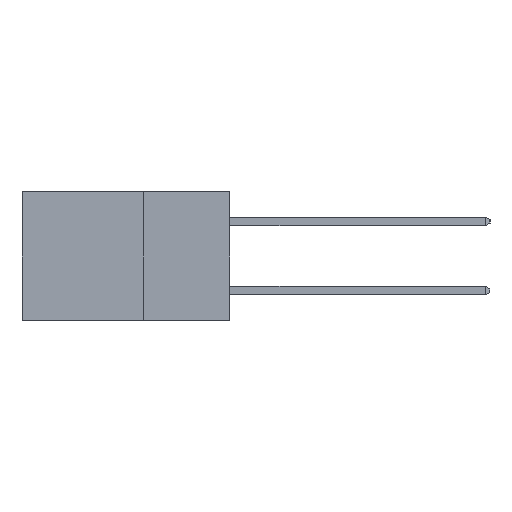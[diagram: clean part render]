
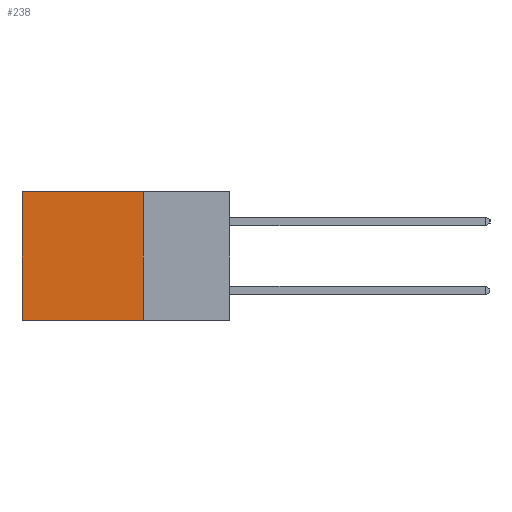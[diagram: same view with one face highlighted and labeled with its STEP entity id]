
A CAD part, left-side view. The second image highlights one B-rep face of the part: STEP entity #238.
In plain terms, the highlighted planar face has unit normal (-1, 0, 0).
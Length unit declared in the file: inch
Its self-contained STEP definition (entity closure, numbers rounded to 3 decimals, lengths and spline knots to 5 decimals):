
#225 = CARTESIAN_POINT ( 'NONE',  ( 0.2615, 0.6, 0. ) ) ;
#238 = ADVANCED_FACE ( 'NONE', ( #16802 ), #2376, .F. ) ;
#592 = EDGE_LOOP ( 'NONE', ( #1698, #6670, #17751, #2903 ) ) ;
#1108 = VERTEX_POINT ( 'NONE', #20829 ) ;
#1698 = ORIENTED_EDGE ( 'NONE', *, *, #1794, .T. ) ;
#1794 = EDGE_CURVE ( 'NONE', #5043, #1108, #2281, .T. ) ;
#2139 = CARTESIAN_POINT ( 'NONE',  ( 0.2615, 0.25, -0.37 ) ) ;
#2281 = LINE ( 'NONE', #13467, #14678 ) ;
#2376 = PLANE ( 'NONE',  #7934 ) ;
#2903 = ORIENTED_EDGE ( 'NONE', *, *, #13747, .T. ) ;
#2960 = VERTEX_POINT ( 'NONE', #21977 ) ;
#3780 = LINE ( 'NONE', #16785, #16598 ) ;
#3852 = DIRECTION ( 'NONE',  ( 0., 0., -1. ) ) ;
#3975 = DIRECTION ( 'NONE',  ( 1., 0., 0. ) ) ;
#4105 = CARTESIAN_POINT ( 'NONE',  ( 0.2615, 0.25, -0.37 ) ) ;
#5010 = CARTESIAN_POINT ( 'NONE',  ( 0.2615, 0.25, 0. ) ) ;
#5043 = VERTEX_POINT ( 'NONE', #225 ) ;
#5943 = EDGE_CURVE ( 'NONE', #8184, #2960, #9927, .T. ) ;
#6011 = VECTOR ( 'NONE', #15779, 39.37008 ) ;
#6670 = ORIENTED_EDGE ( 'NONE', *, *, #20463, .F. ) ;
#7934 = AXIS2_PLACEMENT_3D ( 'NONE', #2139, #3975, #3852 ) ;
#8178 = DIRECTION ( 'NONE',  ( 0., 0., -1. ) ) ;
#8184 = VERTEX_POINT ( 'NONE', #5010 ) ;
#9927 = LINE ( 'NONE', #4105, #18583 ) ;
#11282 = LINE ( 'NONE', #19183, #6011 ) ;
#13347 = DIRECTION ( 'NONE',  ( 0., 1., 0. ) ) ;
#13467 = CARTESIAN_POINT ( 'NONE',  ( 0.2615, 0.6, -0.37 ) ) ;
#13747 = EDGE_CURVE ( 'NONE', #8184, #5043, #11282, .T. ) ;
#14678 = VECTOR ( 'NONE', #8178, 39.37008 ) ;
#15779 = DIRECTION ( 'NONE',  ( 0., 1., 0. ) ) ;
#16598 = VECTOR ( 'NONE', #13347, 39.37008 ) ;
#16785 = CARTESIAN_POINT ( 'NONE',  ( 0.2615, 0.25, -0.37 ) ) ;
#16802 = FACE_OUTER_BOUND ( 'NONE', #592, .T. ) ;
#17751 = ORIENTED_EDGE ( 'NONE', *, *, #5943, .F. ) ;
#18055 = DIRECTION ( 'NONE',  ( 0., 0., -1. ) ) ;
#18583 = VECTOR ( 'NONE', #18055, 39.37008 ) ;
#19183 = CARTESIAN_POINT ( 'NONE',  ( 0.2615, 0.25, 0. ) ) ;
#20463 = EDGE_CURVE ( 'NONE', #2960, #1108, #3780, .T. ) ;
#20829 = CARTESIAN_POINT ( 'NONE',  ( 0.2615, 0.6, -0.37 ) ) ;
#21977 = CARTESIAN_POINT ( 'NONE',  ( 0.2615, 0.25, -0.37 ) ) ;
